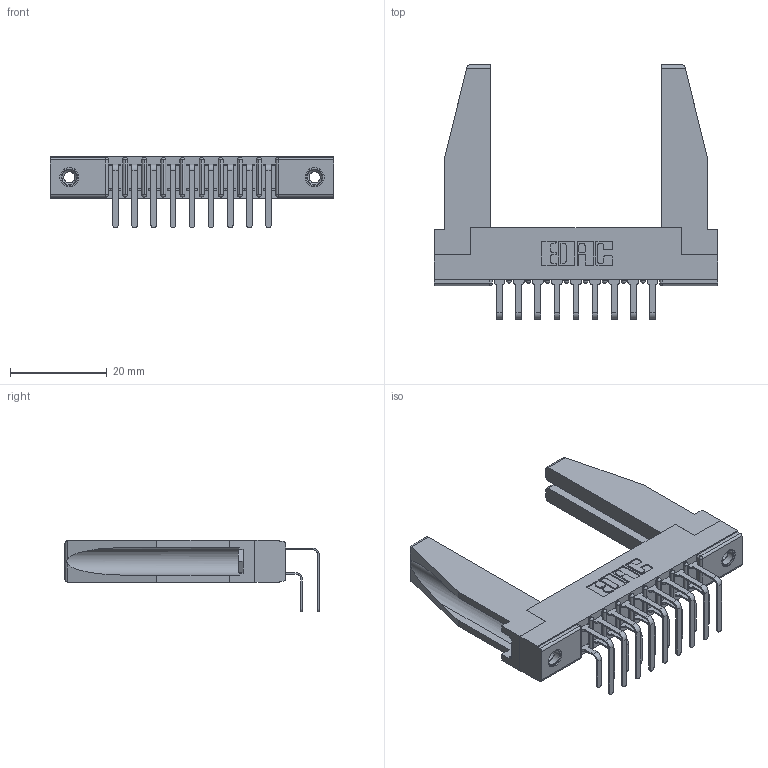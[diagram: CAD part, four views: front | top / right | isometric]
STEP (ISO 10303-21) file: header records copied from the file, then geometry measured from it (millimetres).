
FILE_DESCRIPTION (( 'STEP AP203' ), '1' );
FILE_NAME ('307-018-558-278.STEP', '2019-09-05T20:14:22', ( '' ), ( '' ), 'SwSTEP 2.0', 'SolidWorks 2016', '' );
FILE_SCHEMA (( 'CONFIG_CONTROL_DESIGN' ));
Length unit declared in the file: inch
Products named in the file (6): 345-250-001_345-250-001-102; 307-018-558-278; 307-290-001_558 559 - 1 (Single); 307-220-078; 307 Part_.156 Dia Mounting Holes; 307-290-001_558 - 2 (Single)
Assembly tree (23 placements, depth 2):
  307-018-558-278
    307 Part_.156 Dia Mounting Holes
    307-290-001_558 559 - 1 (Single)  x9
    307-290-001_558 - 2 (Single)  x9
    307-220-078  x2
    345-250-001_345-250-001-102  x2
Bounding box: 58.67 x 52.67 x 14.81 mm (x, y, z)
Volume: 7912.5 mm3; surface area: 10517.5 mm2
Topology: 23 solids, 23 shells, 1158 faces, 3209 edges, 2078 vertices
Faces by surface type: plane 748, cylinder 374, sphere 20, cone 12, torus 4
Entity records: 15958 total; most frequent: CARTESIAN_POINT 2633, ORIENTED_EDGE 2564, DIRECTION 2546, EDGE_CURVE 1282, VECTOR 972, LINE 972, VERTEX_POINT 832, AXIS2_PLACEMENT_3D 787
